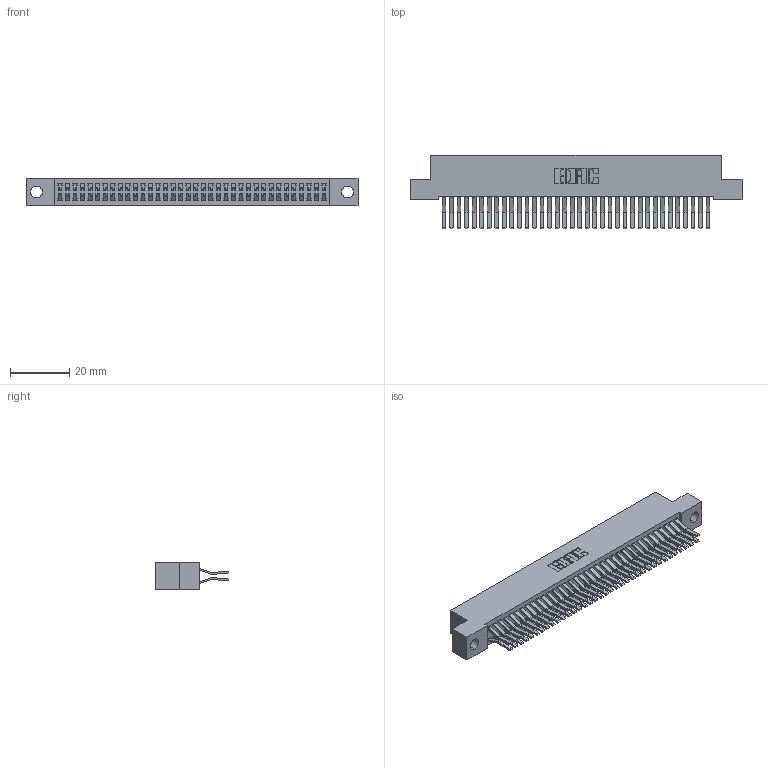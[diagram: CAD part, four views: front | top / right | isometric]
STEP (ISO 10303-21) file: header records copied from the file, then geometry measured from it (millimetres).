
FILE_DESCRIPTION (( 'STEP AP203' ), '1' );
FILE_NAME ('342-072-560-204.STEP', '2018-08-13T10:50:55', ( '' ), ( '' ), 'SwSTEP 2.0', 'SolidWorks 2016', '' );
FILE_SCHEMA (( 'CONFIG_CONTROL_DESIGN' ));
Length unit declared in the file: inch
Products named in the file (3): 345-292-001_560 Tail; 342-072-560-204; 342 Part_.156 TH
Assembly tree (73 placements, depth 2):
  342-072-560-204
    342 Part_.156 TH
    345-292-001_560 Tail  x72
Bounding box: 111.76 x 24.78 x 9.4 mm (x, y, z)
Volume: 10398.9 mm3; surface area: 17736.6 mm2
Topology: 73 solids, 73 shells, 3998 faces, 11891 edges, 7830 vertices
Faces by surface type: plane 2658, cylinder 1340
Entity records: 23895 total; most frequent: CARTESIAN_POINT 3966, ORIENTED_EDGE 3902, DIRECTION 3403, EDGE_CURVE 1951, VECTOR 1819, LINE 1819, VERTEX_POINT 1298, AXIS2_PLACEMENT_3D 792
